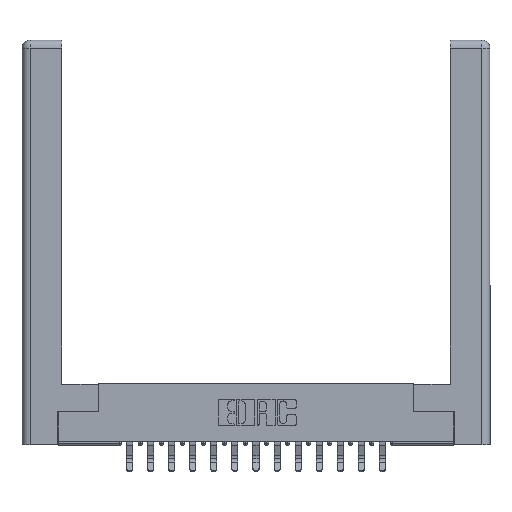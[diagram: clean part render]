
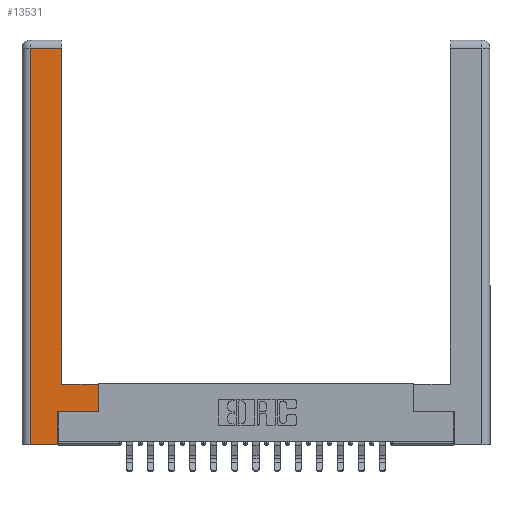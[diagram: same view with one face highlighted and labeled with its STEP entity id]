
A CAD part, top view. The second image highlights one B-rep face of the part: STEP entity #13531.
In plain terms, the highlighted planar face has unit normal (0, 0, 1).
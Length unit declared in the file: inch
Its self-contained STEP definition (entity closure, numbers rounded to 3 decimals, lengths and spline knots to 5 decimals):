
#85 = DIRECTION ( 'NONE',  ( 0., 1., 0. ) ) ;
#117 = VECTOR ( 'NONE', #6806, 39.37008 ) ;
#169 = DIRECTION ( 'NONE',  ( -1., 0., 0. ) ) ;
#1419 = DIRECTION ( 'NONE',  ( -1., 0., 0. ) ) ;
#1436 = DIRECTION ( 'NONE',  ( 1., 0., 0. ) ) ;
#1630 = CARTESIAN_POINT ( 'NONE',  ( 0.565, 0.245, 0. ) ) ;
#2048 = VERTEX_POINT ( 'NONE', #14758 ) ;
#2404 = CARTESIAN_POINT ( 'NONE',  ( 0.265, 0., 0. ) ) ;
#2481 = VERTEX_POINT ( 'NONE', #18453 ) ;
#2687 = CARTESIAN_POINT ( 'NONE',  ( 0.0615, 0., 0. ) ) ;
#2742 = CARTESIAN_POINT ( 'NONE',  ( 0.265, 0., 0. ) ) ;
#2797 = LINE ( 'NONE', #9839, #117 ) ;
#3006 = CARTESIAN_POINT ( 'NONE',  ( 0.0615, 0., 0. ) ) ;
#3215 = VERTEX_POINT ( 'NONE', #4801 ) ;
#3249 = CARTESIAN_POINT ( 'NONE',  ( 0., 0., 0. ) ) ;
#3527 = CARTESIAN_POINT ( 'NONE',  ( 0.295, 3., 0. ) ) ;
#3615 = VERTEX_POINT ( 'NONE', #17253 ) ;
#3857 = EDGE_CURVE ( 'NONE', #13872, #2048, #7538, .T. ) ;
#4040 = FACE_OUTER_BOUND ( 'NONE', #10425, .T. ) ;
#4318 = EDGE_CURVE ( 'NONE', #3615, #14484, #10226, .T. ) ;
#4574 = PLANE ( 'NONE',  #16423 ) ;
#4801 = CARTESIAN_POINT ( 'NONE',  ( 0.0615, 2.94, 0. ) ) ;
#4848 = DIRECTION ( 'NONE',  ( 0., 0., -1. ) ) ;
#5913 = EDGE_CURVE ( 'NONE', #16629, #15770, #11909, .T. ) ;
#6003 = ORIENTED_EDGE ( 'NONE', *, *, #4318, .T. ) ;
#6219 = ORIENTED_EDGE ( 'NONE', *, *, #11029, .T. ) ;
#6427 = LINE ( 'NONE', #2687, #16832 ) ;
#6806 = DIRECTION ( 'NONE',  ( 0., 1., 0. ) ) ;
#7017 = VECTOR ( 'NONE', #85, 39.37008 ) ;
#7267 = LINE ( 'NONE', #9541, #7017 ) ;
#7538 = LINE ( 'NONE', #3527, #18194 ) ;
#7754 = LINE ( 'NONE', #12272, #16449 ) ;
#8296 = DIRECTION ( 'NONE',  ( 0., 1., 0. ) ) ;
#9541 = CARTESIAN_POINT ( 'NONE',  ( 0.565, 0.45, 0. ) ) ;
#9839 = CARTESIAN_POINT ( 'NONE',  ( 0.265, 0.245, 0. ) ) ;
#9845 = ORIENTED_EDGE ( 'NONE', *, *, #3857, .T. ) ;
#10226 = LINE ( 'NONE', #10931, #14959 ) ;
#10331 = VECTOR ( 'NONE', #1419, 39.37008 ) ;
#10425 = EDGE_LOOP ( 'NONE', ( #9845, #6219, #16221, #17865, #12520, #6003, #18025, #19891 ) ) ;
#10737 = DIRECTION ( 'NONE',  ( 1., 0., 0. ) ) ;
#10931 = CARTESIAN_POINT ( 'NONE',  ( 0.565, 0.245, 0. ) ) ;
#11029 = EDGE_CURVE ( 'NONE', #2048, #3215, #14797, .T. ) ;
#11909 = LINE ( 'NONE', #2742, #20047 ) ;
#12272 = CARTESIAN_POINT ( 'NONE',  ( 0.295, 0.45, 0. ) ) ;
#12520 = ORIENTED_EDGE ( 'NONE', *, *, #17278, .T. ) ;
#12834 = EDGE_CURVE ( 'NONE', #2481, #13872, #7754, .T. ) ;
#13531 = ADVANCED_FACE ( 'NONE', ( #4040 ), #4574, .F. ) ;
#13872 = VERTEX_POINT ( 'NONE', #14493 ) ;
#14484 = VERTEX_POINT ( 'NONE', #1630 ) ;
#14493 = CARTESIAN_POINT ( 'NONE',  ( 0.295, 0.45, 0. ) ) ;
#14758 = CARTESIAN_POINT ( 'NONE',  ( 0.295, 2.94, 0. ) ) ;
#14797 = LINE ( 'NONE', #18709, #10331 ) ;
#14959 = VECTOR ( 'NONE', #1436, 39.37008 ) ;
#15770 = VERTEX_POINT ( 'NONE', #2404 ) ;
#16221 = ORIENTED_EDGE ( 'NONE', *, *, #20051, .T. ) ;
#16423 = AXIS2_PLACEMENT_3D ( 'NONE', #3249, #4848, #18887 ) ;
#16449 = VECTOR ( 'NONE', #169, 39.37008 ) ;
#16629 = VERTEX_POINT ( 'NONE', #3006 ) ;
#16832 = VECTOR ( 'NONE', #16900, 39.37008 ) ;
#16900 = DIRECTION ( 'NONE',  ( 0., -1., 0. ) ) ;
#17253 = CARTESIAN_POINT ( 'NONE',  ( 0.265, 0.245, 0. ) ) ;
#17278 = EDGE_CURVE ( 'NONE', #15770, #3615, #2797, .T. ) ;
#17691 = EDGE_CURVE ( 'NONE', #14484, #2481, #7267, .T. ) ;
#17865 = ORIENTED_EDGE ( 'NONE', *, *, #5913, .T. ) ;
#18025 = ORIENTED_EDGE ( 'NONE', *, *, #17691, .T. ) ;
#18194 = VECTOR ( 'NONE', #8296, 39.37008 ) ;
#18453 = CARTESIAN_POINT ( 'NONE',  ( 0.565, 0.45, 0. ) ) ;
#18709 = CARTESIAN_POINT ( 'NONE',  ( 0.0615, 2.94, 0. ) ) ;
#18887 = DIRECTION ( 'NONE',  ( -1., 0., 0. ) ) ;
#19891 = ORIENTED_EDGE ( 'NONE', *, *, #12834, .T. ) ;
#20047 = VECTOR ( 'NONE', #10737, 39.37008 ) ;
#20051 = EDGE_CURVE ( 'NONE', #3215, #16629, #6427, .T. ) ;
